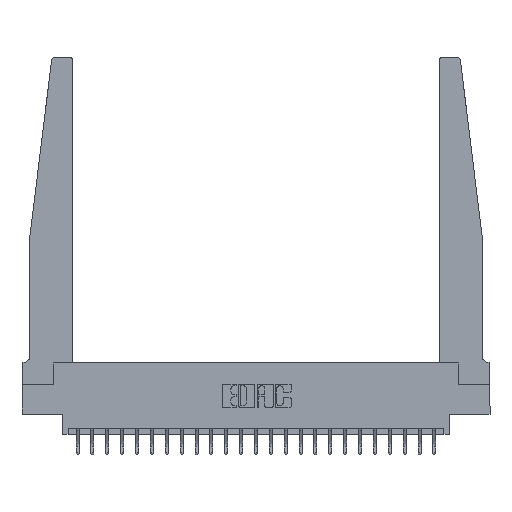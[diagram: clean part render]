
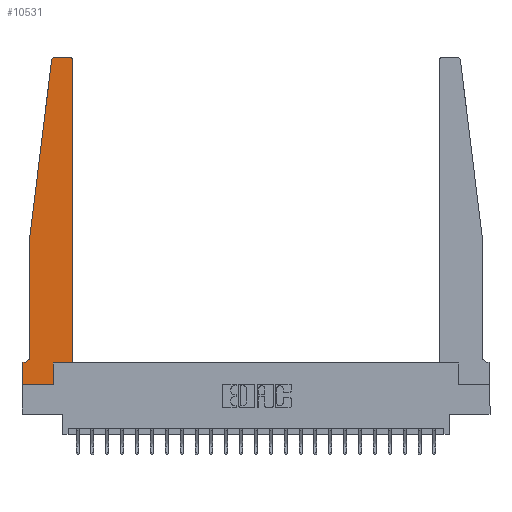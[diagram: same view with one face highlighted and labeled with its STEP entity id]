
A CAD part, top view. The second image highlights one B-rep face of the part: STEP entity #10531.
In plain terms, the highlighted planar face has unit normal (0, 0, 1).
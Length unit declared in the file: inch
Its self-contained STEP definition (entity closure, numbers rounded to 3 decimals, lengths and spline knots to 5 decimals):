
#246 = VERTEX_POINT ( 'NONE', #19879 ) ;
#504 = LINE ( 'NONE', #8086, #2581 ) ;
#684 = DIRECTION ( 'NONE',  ( 1., 0., 0. ) ) ;
#753 = VERTEX_POINT ( 'NONE', #18010 ) ;
#859 = CARTESIAN_POINT ( 'NONE',  ( 0.015, 0.1875, 0.37 ) ) ;
#1044 = CARTESIAN_POINT ( 'NONE',  ( 0.065, 0.2375, 0.37 ) ) ;
#1378 = VECTOR ( 'NONE', #6776, 39.37008 ) ;
#1488 = ORIENTED_EDGE ( 'NONE', *, *, #18365, .T. ) ;
#1705 = VECTOR ( 'NONE', #12691, 39.37008 ) ;
#1991 = DIRECTION ( 'NONE',  ( -1., 0., 0. ) ) ;
#2071 = VERTEX_POINT ( 'NONE', #1044 ) ;
#2076 = DIRECTION ( 'NONE',  ( -0.122, -0.992, 0. ) ) ;
#2251 = DIRECTION ( 'NONE',  ( 0., 0., 1. ) ) ;
#2419 = ORIENTED_EDGE ( 'NONE', *, *, #2954, .T. ) ;
#2581 = VECTOR ( 'NONE', #8209, 39.37008 ) ;
#2600 = DIRECTION ( 'NONE',  ( -1., 0., 0. ) ) ;
#2755 = VECTOR ( 'NONE', #6467, 39.37008 ) ;
#2954 = EDGE_CURVE ( 'NONE', #17821, #753, #16243, .T. ) ;
#2975 = EDGE_CURVE ( 'NONE', #246, #6026, #23964, .T. ) ;
#3063 = CARTESIAN_POINT ( 'NONE',  ( 0.425, 0.18, 0.37 ) ) ;
#3297 = DIRECTION ( 'NONE',  ( 1., 0., 0. ) ) ;
#3707 = DIRECTION ( 'NONE',  ( 0., 0., -1. ) ) ;
#3913 = AXIS2_PLACEMENT_3D ( 'NONE', #19949, #19842, #5060 ) ;
#4239 = VECTOR ( 'NONE', #2600, 39.37008 ) ;
#4301 = AXIS2_PLACEMENT_3D ( 'NONE', #16408, #3707, #1991 ) ;
#4358 = CARTESIAN_POINT ( 'NONE',  ( 0.395, 2.72, 0.37 ) ) ;
#4490 = ORIENTED_EDGE ( 'NONE', *, *, #9061, .T. ) ;
#4840 = VECTOR ( 'NONE', #3297, 39.37008 ) ;
#5060 = DIRECTION ( 'NONE',  ( 1., 0., 0. ) ) ;
#5778 = VERTEX_POINT ( 'NONE', #7403 ) ;
#6026 = VERTEX_POINT ( 'NONE', #21186 ) ;
#6263 = CARTESIAN_POINT ( 'NONE',  ( 0.25, 2.75, 0.37 ) ) ;
#6467 = DIRECTION ( 'NONE',  ( 0., 1., 0. ) ) ;
#6776 = DIRECTION ( 'NONE',  ( 0., -1., 0. ) ) ;
#6957 = CARTESIAN_POINT ( 'NONE',  ( 0., 0., 0.37 ) ) ;
#7318 = DIRECTION ( 'NONE',  ( 0., 1., 0. ) ) ;
#7403 = CARTESIAN_POINT ( 'NONE',  ( 0.065, 1.25, 0.37 ) ) ;
#8086 = CARTESIAN_POINT ( 'NONE',  ( 0.065, 0.1875, 0.37 ) ) ;
#8105 = LINE ( 'NONE', #6263, #4239 ) ;
#8199 = CIRCLE ( 'NONE', #4301, 0.05 ) ;
#8209 = DIRECTION ( 'NONE',  ( -1., 0., 0. ) ) ;
#8413 = AXIS2_PLACEMENT_3D ( 'NONE', #24154, #2251, #22297 ) ;
#8423 = EDGE_CURVE ( 'NONE', #6026, #16318, #16589, .T. ) ;
#8558 = ORIENTED_EDGE ( 'NONE', *, *, #9149, .T. ) ;
#8858 = LINE ( 'NONE', #10794, #1378 ) ;
#9061 = EDGE_CURVE ( 'NONE', #753, #12165, #9849, .T. ) ;
#9149 = EDGE_CURVE ( 'NONE', #16318, #15664, #22087, .T. ) ;
#9160 = ORIENTED_EDGE ( 'NONE', *, *, #18448, .T. ) ;
#9813 = ORIENTED_EDGE ( 'NONE', *, *, #17680, .T. ) ;
#9849 = LINE ( 'NONE', #15829, #16607 ) ;
#10097 = DIRECTION ( 'NONE',  ( 1., 0., 0. ) ) ;
#10404 = EDGE_CURVE ( 'NONE', #5778, #2071, #8858, .T. ) ;
#10531 = ADVANCED_FACE ( 'NONE', ( #17154 ), #16902, .T. ) ;
#10794 = CARTESIAN_POINT ( 'NONE',  ( 0.065, 1.25, 0.37 ) ) ;
#10957 = VERTEX_POINT ( 'NONE', #20311 ) ;
#11156 = EDGE_CURVE ( 'NONE', #14798, #17821, #504, .T. ) ;
#11357 = LINE ( 'NONE', #18828, #18361 ) ;
#11956 = LINE ( 'NONE', #19297, #2755 ) ;
#12108 = ORIENTED_EDGE ( 'NONE', *, *, #11156, .T. ) ;
#12165 = VERTEX_POINT ( 'NONE', #14009 ) ;
#12691 = DIRECTION ( 'NONE',  ( 0., -1., 0. ) ) ;
#13146 = CARTESIAN_POINT ( 'NONE',  ( 0.24675, 2.72367, 0.37 ) ) ;
#13319 = EDGE_CURVE ( 'NONE', #15664, #10957, #8105, .T. ) ;
#13531 = AXIS2_PLACEMENT_3D ( 'NONE', #4358, #17410, #684 ) ;
#14009 = CARTESIAN_POINT ( 'NONE',  ( 0.2605, 0., 0.37 ) ) ;
#14798 = VERTEX_POINT ( 'NONE', #859 ) ;
#14960 = ORIENTED_EDGE ( 'NONE', *, *, #2975, .T. ) ;
#15664 = VERTEX_POINT ( 'NONE', #16067 ) ;
#15829 = CARTESIAN_POINT ( 'NONE',  ( 0., 0., 0.37 ) ) ;
#16067 = CARTESIAN_POINT ( 'NONE',  ( 0.395, 2.75, 0.37 ) ) ;
#16243 = LINE ( 'NONE', #6957, #1705 ) ;
#16318 = VERTEX_POINT ( 'NONE', #19010 ) ;
#16408 = CARTESIAN_POINT ( 'NONE',  ( 0.015, 0.2375, 0.37 ) ) ;
#16460 = CARTESIAN_POINT ( 'NONE',  ( 0.425, 0.18, 0.37 ) ) ;
#16589 = LINE ( 'NONE', #16460, #22856 ) ;
#16607 = VECTOR ( 'NONE', #10097, 39.37008 ) ;
#16902 = PLANE ( 'NONE',  #8413 ) ;
#17154 = FACE_OUTER_BOUND ( 'NONE', #17599, .T. ) ;
#17410 = DIRECTION ( 'NONE',  ( 0., 0., 1. ) ) ;
#17420 = VERTEX_POINT ( 'NONE', #13146 ) ;
#17599 = EDGE_LOOP ( 'NONE', ( #19655, #9813, #1488, #17851, #23481, #12108, #2419, #4490, #9160, #14960, #20164, #8558 ) ) ;
#17680 = EDGE_CURVE ( 'NONE', #10957, #17420, #18345, .T. ) ;
#17814 = EDGE_CURVE ( 'NONE', #2071, #14798, #8199, .T. ) ;
#17821 = VERTEX_POINT ( 'NONE', #20193 ) ;
#17851 = ORIENTED_EDGE ( 'NONE', *, *, #10404, .T. ) ;
#18010 = CARTESIAN_POINT ( 'NONE',  ( 0., 0., 0.37 ) ) ;
#18345 = CIRCLE ( 'NONE', #3913, 0.03 ) ;
#18361 = VECTOR ( 'NONE', #2076, 39.37008 ) ;
#18365 = EDGE_CURVE ( 'NONE', #17420, #5778, #11357, .T. ) ;
#18448 = EDGE_CURVE ( 'NONE', #12165, #246, #11956, .T. ) ;
#18828 = CARTESIAN_POINT ( 'NONE',  ( 0.065, 1.25, 0.37 ) ) ;
#19010 = CARTESIAN_POINT ( 'NONE',  ( 0.425, 2.72, 0.37 ) ) ;
#19297 = CARTESIAN_POINT ( 'NONE',  ( 0.2605, 0.18, 0.37 ) ) ;
#19655 = ORIENTED_EDGE ( 'NONE', *, *, #13319, .T. ) ;
#19842 = DIRECTION ( 'NONE',  ( 0., 0., 1. ) ) ;
#19879 = CARTESIAN_POINT ( 'NONE',  ( 0.2605, 0.18, 0.37 ) ) ;
#19949 = CARTESIAN_POINT ( 'NONE',  ( 0.27653, 2.72, 0.37 ) ) ;
#20164 = ORIENTED_EDGE ( 'NONE', *, *, #8423, .T. ) ;
#20193 = CARTESIAN_POINT ( 'NONE',  ( 0., 0.1875, 0.37 ) ) ;
#20311 = CARTESIAN_POINT ( 'NONE',  ( 0.27653, 2.75, 0.37 ) ) ;
#21186 = CARTESIAN_POINT ( 'NONE',  ( 0.425, 0.18, 0.37 ) ) ;
#22087 = CIRCLE ( 'NONE', #13531, 0.03 ) ;
#22297 = DIRECTION ( 'NONE',  ( 1., 0., 0. ) ) ;
#22856 = VECTOR ( 'NONE', #7318, 39.37008 ) ;
#23481 = ORIENTED_EDGE ( 'NONE', *, *, #17814, .T. ) ;
#23964 = LINE ( 'NONE', #3063, #4840 ) ;
#24154 = CARTESIAN_POINT ( 'NONE',  ( 0., 0.1875, 0.37 ) ) ;
